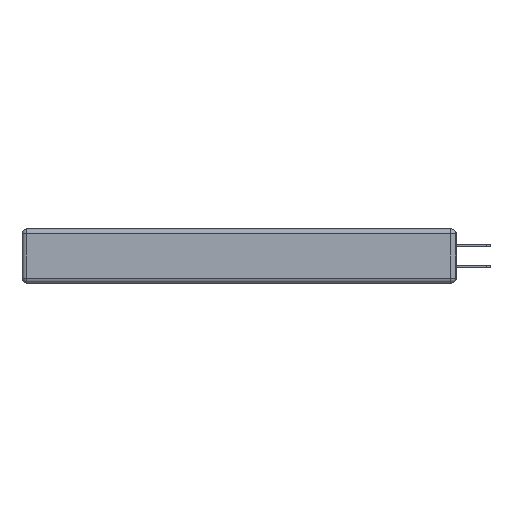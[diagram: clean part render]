
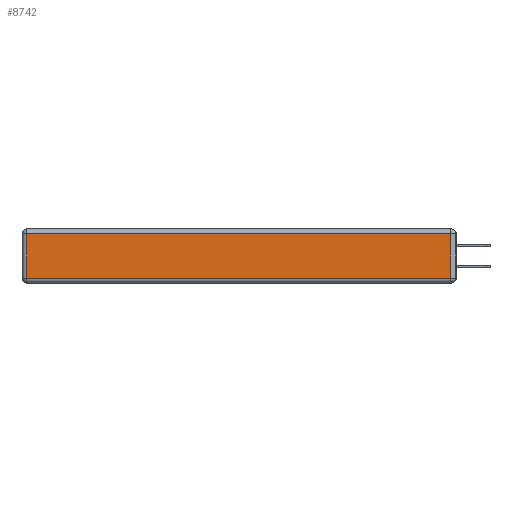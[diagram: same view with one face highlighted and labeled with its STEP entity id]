
A CAD part, left-side view. The second image highlights one B-rep face of the part: STEP entity #8742.
In plain terms, the highlighted planar face has unit normal (-1, 0, 0).
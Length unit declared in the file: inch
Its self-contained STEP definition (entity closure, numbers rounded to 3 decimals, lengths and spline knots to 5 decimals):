
#1798 = CARTESIAN_POINT ( 'NONE',  ( 0., 0., -0.313 ) ) ;
#2198 = VERTEX_POINT ( 'NONE', #15850 ) ;
#3068 = VECTOR ( 'NONE', #3836, 39.37008 ) ;
#3321 = VERTEX_POINT ( 'NONE', #11803 ) ;
#3836 = DIRECTION ( 'NONE',  ( 0., 1., 0. ) ) ;
#3903 = VECTOR ( 'NONE', #14667, 39.37008 ) ;
#4442 = VERTEX_POINT ( 'NONE', #14401 ) ;
#4541 = LINE ( 'NONE', #1798, #16546 ) ;
#4791 = VERTEX_POINT ( 'NONE', #5503 ) ;
#5015 = EDGE_CURVE ( 'NONE', #4442, #4791, #11243, .T. ) ;
#5030 = DIRECTION ( 'NONE',  ( 0., 0., -1. ) ) ;
#5503 = CARTESIAN_POINT ( 'NONE',  ( 0., 0.03, -0.03 ) ) ;
#5999 = ORIENTED_EDGE ( 'NONE', *, *, #10536, .T. ) ;
#8279 = PLANE ( 'NONE',  #15945 ) ;
#8742 = ADVANCED_FACE ( 'NONE', ( #18475 ), #8279, .T. ) ;
#8826 = ORIENTED_EDGE ( 'NONE', *, *, #10736, .T. ) ;
#9570 = ORIENTED_EDGE ( 'NONE', *, *, #10764, .T. ) ;
#9828 = DIRECTION ( 'NONE',  ( 0., -1., 0. ) ) ;
#9842 = CARTESIAN_POINT ( 'NONE',  ( 0., 0., -0.343 ) ) ;
#10264 = DIRECTION ( 'NONE',  ( 0., 0., 1. ) ) ;
#10536 = EDGE_CURVE ( 'NONE', #4791, #3321, #19726, .T. ) ;
#10736 = EDGE_CURVE ( 'NONE', #3321, #2198, #15072, .T. ) ;
#10764 = EDGE_CURVE ( 'NONE', #2198, #4442, #4541, .T. ) ;
#11243 = LINE ( 'NONE', #13201, #3903 ) ;
#11401 = ORIENTED_EDGE ( 'NONE', *, *, #5015, .T. ) ;
#11803 = CARTESIAN_POINT ( 'NONE',  ( 0., 2.72, -0.03 ) ) ;
#13184 = DIRECTION ( 'NONE',  ( -1., 0., 0. ) ) ;
#13201 = CARTESIAN_POINT ( 'NONE',  ( 0., 0.03, -0.343 ) ) ;
#14401 = CARTESIAN_POINT ( 'NONE',  ( 0., 0.03, -0.313 ) ) ;
#14667 = DIRECTION ( 'NONE',  ( 0., 0., 1. ) ) ;
#15072 = LINE ( 'NONE', #15844, #18726 ) ;
#15844 = CARTESIAN_POINT ( 'NONE',  ( 0., 2.72, -0.343 ) ) ;
#15850 = CARTESIAN_POINT ( 'NONE',  ( 0., 2.72, -0.313 ) ) ;
#15945 = AXIS2_PLACEMENT_3D ( 'NONE', #9842, #13184, #10264 ) ;
#16546 = VECTOR ( 'NONE', #9828, 39.37008 ) ;
#17623 = EDGE_LOOP ( 'NONE', ( #9570, #11401, #5999, #8826 ) ) ;
#18475 = FACE_OUTER_BOUND ( 'NONE', #17623, .T. ) ;
#18726 = VECTOR ( 'NONE', #5030, 39.37008 ) ;
#19022 = CARTESIAN_POINT ( 'NONE',  ( 0., 2.75, -0.03 ) ) ;
#19726 = LINE ( 'NONE', #19022, #3068 ) ;
